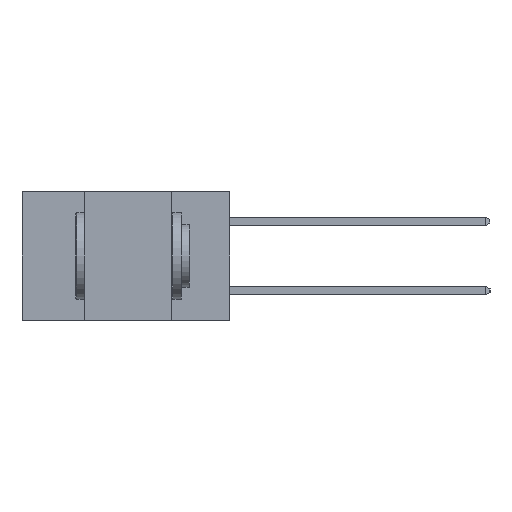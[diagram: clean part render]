
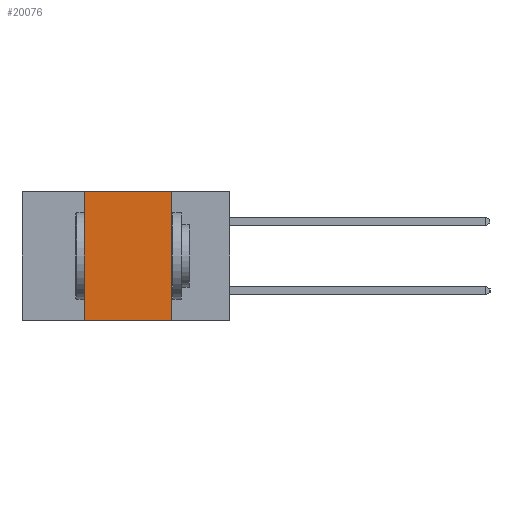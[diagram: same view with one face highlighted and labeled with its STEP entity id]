
A CAD part, left-side view. The second image highlights one B-rep face of the part: STEP entity #20076.
In plain terms, the highlighted planar face has unit normal (-1, 0, 0).
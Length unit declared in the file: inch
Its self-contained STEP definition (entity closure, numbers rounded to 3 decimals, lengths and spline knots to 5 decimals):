
#179 = EDGE_LOOP ( 'NONE', ( #9928, #18507, #18975, #3483 ) ) ;
#495 = DIRECTION ( 'NONE',  ( 0., -1., 0. ) ) ;
#738 = EDGE_CURVE ( 'NONE', #8628, #982, #10372, .T. ) ;
#982 = VERTEX_POINT ( 'NONE', #1028 ) ;
#1028 = CARTESIAN_POINT ( 'NONE',  ( 0., 0.17, 0. ) ) ;
#1480 = DIRECTION ( 'NONE',  ( 0., 0., 1. ) ) ;
#1511 = DIRECTION ( 'NONE',  ( 0., 0., -1. ) ) ;
#1938 = AXIS2_PLACEMENT_3D ( 'NONE', #14084, #11054, #1511 ) ;
#2394 = CARTESIAN_POINT ( 'NONE',  ( 0., 0.42, -0.37 ) ) ;
#2513 = VECTOR ( 'NONE', #495, 39.37008 ) ;
#2807 = VERTEX_POINT ( 'NONE', #8754 ) ;
#2910 = EDGE_CURVE ( 'NONE', #19225, #8628, #4107, .T. ) ;
#2950 = CARTESIAN_POINT ( 'NONE',  ( 0., 0.17, -0.37 ) ) ;
#3032 = LINE ( 'NONE', #17649, #2513 ) ;
#3483 = ORIENTED_EDGE ( 'NONE', *, *, #13837, .T. ) ;
#3604 = VECTOR ( 'NONE', #1480, 39.37008 ) ;
#4107 = LINE ( 'NONE', #2394, #3604 ) ;
#7008 = DIRECTION ( 'NONE',  ( 0., -1., 0. ) ) ;
#7259 = EDGE_CURVE ( 'NONE', #982, #2807, #11158, .T. ) ;
#7554 = VECTOR ( 'NONE', #9421, 39.37008 ) ;
#8628 = VERTEX_POINT ( 'NONE', #10203 ) ;
#8754 = CARTESIAN_POINT ( 'NONE',  ( 0., 0.17, -0.37 ) ) ;
#9421 = DIRECTION ( 'NONE',  ( 0., 0., -1. ) ) ;
#9928 = ORIENTED_EDGE ( 'NONE', *, *, #7259, .F. ) ;
#10203 = CARTESIAN_POINT ( 'NONE',  ( 0., 0.42, 0. ) ) ;
#10372 = LINE ( 'NONE', #15257, #13486 ) ;
#11054 = DIRECTION ( 'NONE',  ( 1., 0., 0. ) ) ;
#11158 = LINE ( 'NONE', #2950, #7554 ) ;
#13486 = VECTOR ( 'NONE', #7008, 39.37008 ) ;
#13837 = EDGE_CURVE ( 'NONE', #19225, #2807, #3032, .T. ) ;
#14084 = CARTESIAN_POINT ( 'NONE',  ( 0., 0.6, 0. ) ) ;
#14428 = FACE_OUTER_BOUND ( 'NONE', #179, .T. ) ;
#15257 = CARTESIAN_POINT ( 'NONE',  ( 0., 0.6, 0. ) ) ;
#16646 = CARTESIAN_POINT ( 'NONE',  ( 0., 0.42, -0.37 ) ) ;
#17649 = CARTESIAN_POINT ( 'NONE',  ( 0., 0.6, -0.37 ) ) ;
#18507 = ORIENTED_EDGE ( 'NONE', *, *, #738, .F. ) ;
#18975 = ORIENTED_EDGE ( 'NONE', *, *, #2910, .F. ) ;
#19225 = VERTEX_POINT ( 'NONE', #16646 ) ;
#20076 = ADVANCED_FACE ( 'NONE', ( #14428 ), #20126, .F. ) ;
#20126 = PLANE ( 'NONE',  #1938 ) ;
